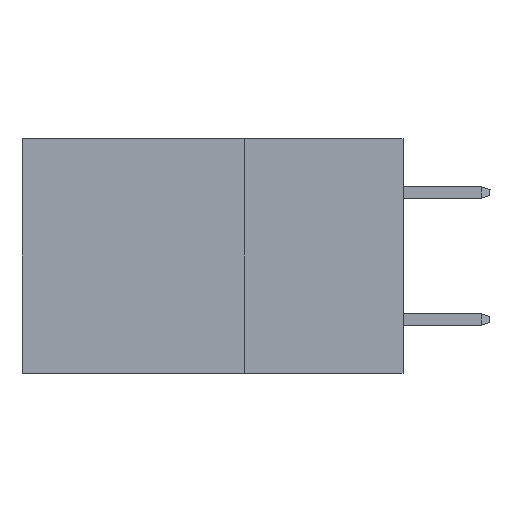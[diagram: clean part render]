
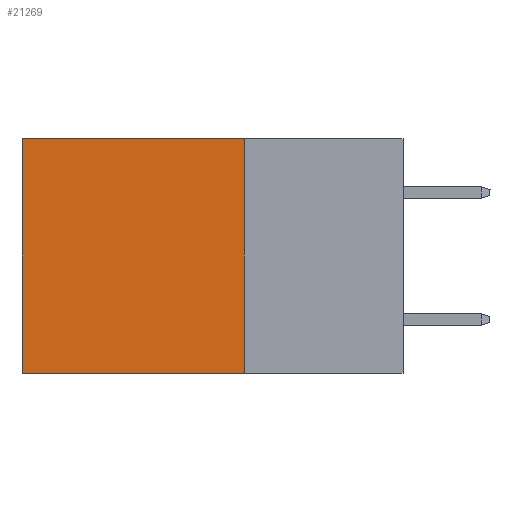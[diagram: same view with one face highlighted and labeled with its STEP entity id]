
A CAD part, left-side view. The second image highlights one B-rep face of the part: STEP entity #21269.
In plain terms, the highlighted planar face has unit normal (-1, 0, 0).
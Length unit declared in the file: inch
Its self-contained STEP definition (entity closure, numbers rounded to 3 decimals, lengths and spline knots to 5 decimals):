
#414 = LINE ( 'NONE', #15045, #34911 ) ;
#1956 = EDGE_CURVE ( 'NONE', #12207, #15792, #35829, .T. ) ;
#8280 = ORIENTED_EDGE ( 'NONE', *, *, #31115, .T. ) ;
#8310 = CARTESIAN_POINT ( 'NONE',  ( 0.2875, 0.6, -0.37 ) ) ;
#9055 = EDGE_CURVE ( 'NONE', #12207, #16636, #17210, .T. ) ;
#9628 = EDGE_LOOP ( 'NONE', ( #8280, #23199, #13196, #30891 ) ) ;
#11351 = CARTESIAN_POINT ( 'NONE',  ( 0.2875, 0.25, -0.37 ) ) ;
#12207 = VERTEX_POINT ( 'NONE', #37116 ) ;
#13196 = ORIENTED_EDGE ( 'NONE', *, *, #1956, .F. ) ;
#14842 = CARTESIAN_POINT ( 'NONE',  ( 0.2875, 0.25, -0.37 ) ) ;
#15045 = CARTESIAN_POINT ( 'NONE',  ( 0.2875, 0.6, 0. ) ) ;
#15416 = AXIS2_PLACEMENT_3D ( 'NONE', #41838, #23126, #30336 ) ;
#15792 = VERTEX_POINT ( 'NONE', #14842 ) ;
#16636 = VERTEX_POINT ( 'NONE', #19674 ) ;
#17210 = LINE ( 'NONE', #39247, #37981 ) ;
#18317 = DIRECTION ( 'NONE',  ( 0., 1., 0. ) ) ;
#19674 = CARTESIAN_POINT ( 'NONE',  ( 0.2875, 0.6, 0. ) ) ;
#21269 = ADVANCED_FACE ( 'NONE', ( #22906 ), #44744, .F. ) ;
#21306 = VERTEX_POINT ( 'NONE', #8310 ) ;
#21877 = LINE ( 'NONE', #11351, #37617 ) ;
#22906 = FACE_OUTER_BOUND ( 'NONE', #9628, .T. ) ;
#23126 = DIRECTION ( 'NONE',  ( 1., 0., 0. ) ) ;
#23199 = ORIENTED_EDGE ( 'NONE', *, *, #45034, .F. ) ;
#28641 = CARTESIAN_POINT ( 'NONE',  ( 0.2875, 0.25, 0. ) ) ;
#29655 = DIRECTION ( 'NONE',  ( 0., 0., -1. ) ) ;
#30336 = DIRECTION ( 'NONE',  ( 0., 0., -1. ) ) ;
#30891 = ORIENTED_EDGE ( 'NONE', *, *, #9055, .T. ) ;
#31115 = EDGE_CURVE ( 'NONE', #16636, #21306, #414, .T. ) ;
#31584 = DIRECTION ( 'NONE',  ( 0., 1., 0. ) ) ;
#32010 = DIRECTION ( 'NONE',  ( 0., 0., -1. ) ) ;
#34911 = VECTOR ( 'NONE', #29655, 39.37008 ) ;
#35829 = LINE ( 'NONE', #28641, #37179 ) ;
#37116 = CARTESIAN_POINT ( 'NONE',  ( 0.2875, 0.25, 0. ) ) ;
#37179 = VECTOR ( 'NONE', #32010, 39.37008 ) ;
#37617 = VECTOR ( 'NONE', #18317, 39.37008 ) ;
#37981 = VECTOR ( 'NONE', #31584, 39.37008 ) ;
#39247 = CARTESIAN_POINT ( 'NONE',  ( 0.2875, 0.25, 0. ) ) ;
#41838 = CARTESIAN_POINT ( 'NONE',  ( 0.2875, 0.25, 0. ) ) ;
#44744 = PLANE ( 'NONE',  #15416 ) ;
#45034 = EDGE_CURVE ( 'NONE', #15792, #21306, #21877, .T. ) ;
